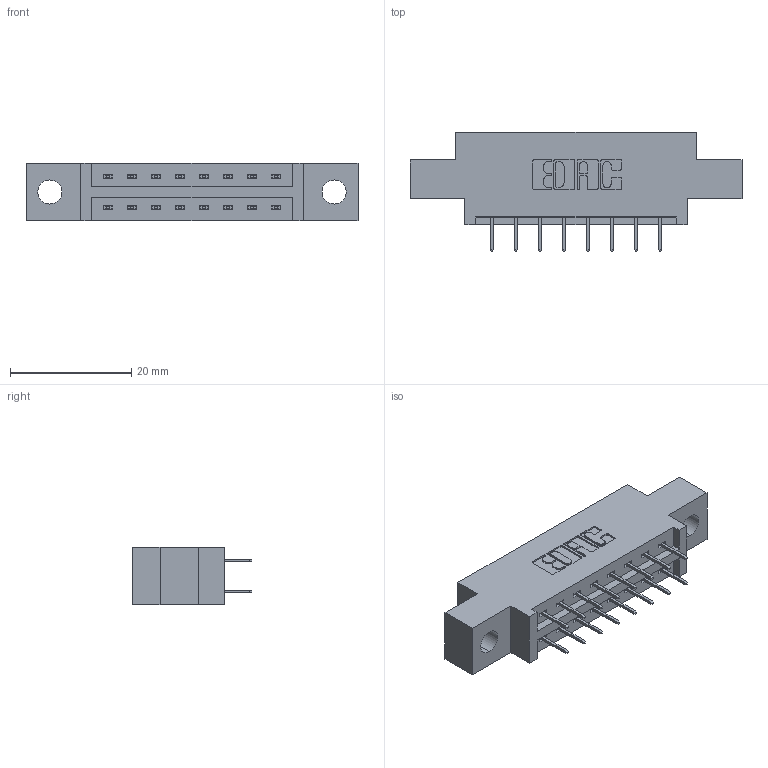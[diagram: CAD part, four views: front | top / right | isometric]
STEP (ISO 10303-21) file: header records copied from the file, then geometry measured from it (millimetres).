
FILE_DESCRIPTION (( 'STEP AP203' ), '1' );
FILE_NAME ('387-016-524-804.STEP', '2018-09-11T10:03:15', ( '' ), ( '' ), 'SwSTEP 2.0', 'SolidWorks 2016', '' );
FILE_SCHEMA (( 'CONFIG_CONTROL_DESIGN' ));
Length unit declared in the file: inch
Products named in the file (3): 337 Part_0.170 Offset - 0.156 Dia-TH; 345-292-001_345-293-124; 387-016-524-804
Assembly tree (17 placements, depth 2):
  387-016-524-804
    337 Part_0.170 Offset - 0.156 Dia-TH
    345-292-001_345-293-124  x16
Bounding box: 54.71 x 19.69 x 9.4 mm (x, y, z)
Volume: 5083.8 mm3; surface area: 5247.2 mm2
Topology: 17 solids, 17 shells, 1046 faces, 2963 edges, 1910 vertices
Faces by surface type: plane 778, cylinder 268
Entity records: 10809 total; most frequent: CARTESIAN_POINT 1850, ORIENTED_EDGE 1786, DIRECTION 1637, EDGE_CURVE 893, LINE 769, VECTOR 769, VERTEX_POINT 590, AXIS2_PLACEMENT_3D 434
